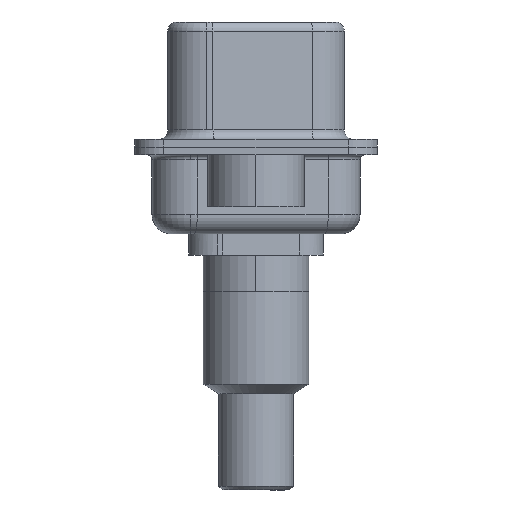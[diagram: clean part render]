
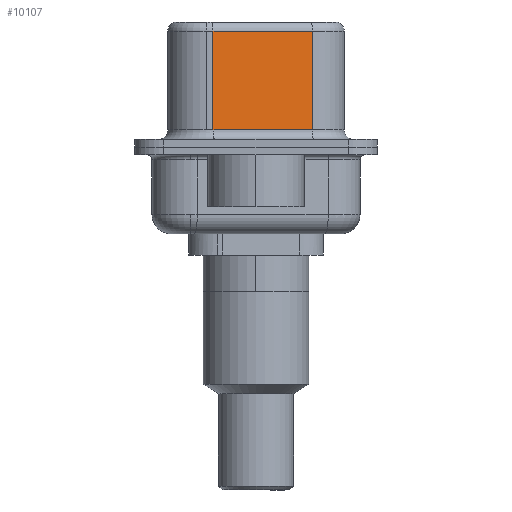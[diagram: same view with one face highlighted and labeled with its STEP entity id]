
A CAD part, left-side view. The second image highlights one B-rep face of the part: STEP entity #10107.
In plain terms, the highlighted planar face has unit normal (-0.985, -0.174, 0).
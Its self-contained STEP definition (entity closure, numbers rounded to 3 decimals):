
#327 = EDGE_CURVE ( 'NONE', #20381, #16828, #20884, .T. ) ;
#780 = LINE ( 'NONE', #17056, #4987 ) ;
#971 = EDGE_CURVE ( 'NONE', #20381, #17316, #12224, .T. ) ;
#975 = EDGE_CURVE ( 'NONE', #17926, #17316, #16106, .T. ) ;
#1478 = CARTESIAN_POINT ( 'NONE',  ( 3.655, 2.233, 0.9 ) ) ;
#1964 = CARTESIAN_POINT ( 'NONE',  ( 4.565, -2.927, 6.02 ) ) ;
#2084 = DIRECTION ( 'NONE',  ( -0.174, 0.985, 0. ) ) ;
#4554 = ORIENTED_EDGE ( 'NONE', *, *, #971, .F. ) ;
#4987 = VECTOR ( 'NONE', #18668, 1000. ) ;
#5518 = FACE_OUTER_BOUND ( 'NONE', #9399, .T. ) ;
#5572 = DIRECTION ( 'NONE',  ( 0.985, 0.174, 0. ) ) ;
#6532 = ORIENTED_EDGE ( 'NONE', *, *, #8766, .T. ) ;
#7140 = CARTESIAN_POINT ( 'NONE',  ( 4.565, -2.927, 6.02 ) ) ;
#8531 = CARTESIAN_POINT ( 'NONE',  ( 3.655, 2.233, 6.02 ) ) ;
#8766 = EDGE_CURVE ( 'NONE', #16828, #17926, #780, .T. ) ;
#9399 = EDGE_LOOP ( 'NONE', ( #4554, #10140, #6532, #20704 ) ) ;
#10107 = ADVANCED_FACE ( 'NONE', ( #5518 ), #10675, .F. ) ;
#10140 = ORIENTED_EDGE ( 'NONE', *, *, #327, .T. ) ;
#10675 = PLANE ( 'NONE',  #21059 ) ;
#10903 = CARTESIAN_POINT ( 'NONE',  ( 4.565, -2.927, 0.9 ) ) ;
#11176 = VECTOR ( 'NONE', #11756, 1000. ) ;
#11338 = DIRECTION ( 'NONE',  ( 0., 0., -1. ) ) ;
#11756 = DIRECTION ( 'NONE',  ( 0.174, -0.985, 0. ) ) ;
#12224 = LINE ( 'NONE', #13771, #19856 ) ;
#12327 = CARTESIAN_POINT ( 'NONE',  ( 4.565, -2.927, 6.52 ) ) ;
#13771 = CARTESIAN_POINT ( 'NONE',  ( 4.565, -2.927, 6.52 ) ) ;
#15093 = DIRECTION ( 'NONE',  ( -0.174, 0.985, 0. ) ) ;
#16106 = LINE ( 'NONE', #10903, #11176 ) ;
#16828 = VERTEX_POINT ( 'NONE', #8531 ) ;
#17056 = CARTESIAN_POINT ( 'NONE',  ( 3.655, 2.233, 6.52 ) ) ;
#17316 = VERTEX_POINT ( 'NONE', #19090 ) ;
#17926 = VERTEX_POINT ( 'NONE', #1478 ) ;
#18668 = DIRECTION ( 'NONE',  ( 0., 0., -1. ) ) ;
#19090 = CARTESIAN_POINT ( 'NONE',  ( 4.565, -2.927, 0.9 ) ) ;
#19856 = VECTOR ( 'NONE', #11338, 1000. ) ;
#19900 = VECTOR ( 'NONE', #15093, 1000. ) ;
#20381 = VERTEX_POINT ( 'NONE', #1964 ) ;
#20704 = ORIENTED_EDGE ( 'NONE', *, *, #975, .T. ) ;
#20884 = LINE ( 'NONE', #7140, #19900 ) ;
#21059 = AXIS2_PLACEMENT_3D ( 'NONE', #12327, #5572, #2084 ) ;
